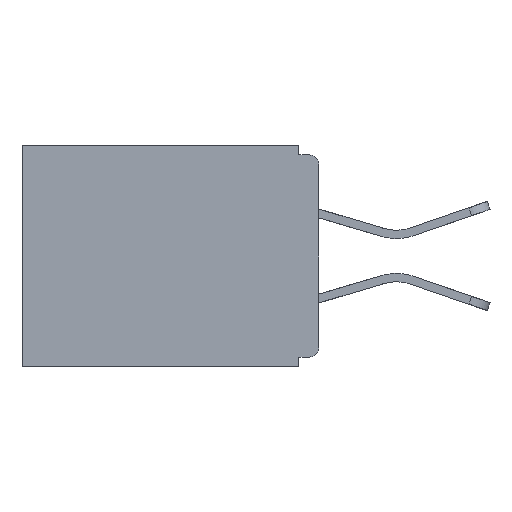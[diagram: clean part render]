
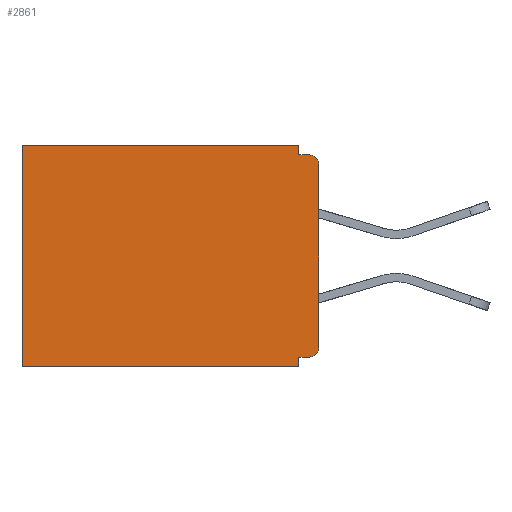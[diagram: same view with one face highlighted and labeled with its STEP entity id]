
A CAD part, left-side view. The second image highlights one B-rep face of the part: STEP entity #2861.
In plain terms, the highlighted planar face has unit normal (-1, 0, 0).
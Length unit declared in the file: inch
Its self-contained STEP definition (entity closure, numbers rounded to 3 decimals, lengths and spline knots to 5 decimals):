
#198 = ORIENTED_EDGE ( 'NONE', *, *, #13432, .T. ) ;
#289 = DIRECTION ( 'NONE',  ( 0., 1., 0. ) ) ;
#593 = AXIS2_PLACEMENT_3D ( 'NONE', #17195, #8387, #11389 ) ;
#1648 = DIRECTION ( 'NONE',  ( 0., 0., -1. ) ) ;
#1740 = ORIENTED_EDGE ( 'NONE', *, *, #16769, .T. ) ;
#2199 = VECTOR ( 'NONE', #4554, 39.37008 ) ;
#2351 = PLANE ( 'NONE',  #15073 ) ;
#2547 = DIRECTION ( 'NONE',  ( 0., 0., -1. ) ) ;
#2598 = EDGE_CURVE ( 'NONE', #16685, #11531, #4499, .T. ) ;
#2722 = ORIENTED_EDGE ( 'NONE', *, *, #9086, .T. ) ;
#2753 = ORIENTED_EDGE ( 'NONE', *, *, #14645, .F. ) ;
#2861 = ADVANCED_FACE ( 'NONE', ( #17775 ), #2351, .F. ) ;
#3551 = EDGE_CURVE ( 'NONE', #8760, #5759, #18661, .T. ) ;
#4011 = VECTOR ( 'NONE', #11175, 39.37008 ) ;
#4232 = EDGE_CURVE ( 'NONE', #6971, #15433, #12115, .T. ) ;
#4321 = VECTOR ( 'NONE', #14092, 39.37008 ) ;
#4493 = CARTESIAN_POINT ( 'NONE',  ( 0.298, 0., -0.328 ) ) ;
#4499 = LINE ( 'NONE', #11701, #15714 ) ;
#4554 = DIRECTION ( 'NONE',  ( 0., -1., 0. ) ) ;
#4942 = CARTESIAN_POINT ( 'NONE',  ( 0.298, 0.46, 0. ) ) ;
#5049 = CARTESIAN_POINT ( 'NONE',  ( 0.298, 0.015, -0.015 ) ) ;
#5377 = CARTESIAN_POINT ( 'NONE',  ( 0.298, 0.031, -0.343 ) ) ;
#5759 = VERTEX_POINT ( 'NONE', #7385 ) ;
#5948 = LINE ( 'NONE', #5377, #7773 ) ;
#6378 = CIRCLE ( 'NONE', #7844, 0.015 ) ;
#6809 = CARTESIAN_POINT ( 'NONE',  ( 0.298, 0., 0. ) ) ;
#6944 = ORIENTED_EDGE ( 'NONE', *, *, #10040, .T. ) ;
#6971 = VERTEX_POINT ( 'NONE', #16929 ) ;
#7042 = ORIENTED_EDGE ( 'NONE', *, *, #14113, .F. ) ;
#7327 = VERTEX_POINT ( 'NONE', #8107 ) ;
#7385 = CARTESIAN_POINT ( 'NONE',  ( 0.298, 0.031, -0.328 ) ) ;
#7593 = CARTESIAN_POINT ( 'NONE',  ( 0.298, 0.46, 0. ) ) ;
#7655 = VECTOR ( 'NONE', #10440, 39.37008 ) ;
#7743 = DIRECTION ( 'NONE',  ( 0., 0., -1. ) ) ;
#7773 = VECTOR ( 'NONE', #8304, 39.37008 ) ;
#7844 = AXIS2_PLACEMENT_3D ( 'NONE', #15994, #16176, #1648 ) ;
#8038 = VECTOR ( 'NONE', #7743, 39.37008 ) ;
#8107 = CARTESIAN_POINT ( 'NONE',  ( 0.298, 0.031, 0. ) ) ;
#8125 = CARTESIAN_POINT ( 'NONE',  ( 0.298, 0., 0. ) ) ;
#8304 = DIRECTION ( 'NONE',  ( 0., 0., -1. ) ) ;
#8387 = DIRECTION ( 'NONE',  ( -1., 0., 0. ) ) ;
#8572 = CARTESIAN_POINT ( 'NONE',  ( 0.298, 0., -0.313 ) ) ;
#8760 = VERTEX_POINT ( 'NONE', #15895 ) ;
#8946 = CARTESIAN_POINT ( 'NONE',  ( 0.298, 0., -0.015 ) ) ;
#9086 = EDGE_CURVE ( 'NONE', #8760, #15433, #6378, .T. ) ;
#9527 = EDGE_LOOP ( 'NONE', ( #6944, #7042, #10122, #198, #1740, #15224, #2753, #11687, #2722, #15324 ) ) ;
#9729 = LINE ( 'NONE', #7593, #7655 ) ;
#9773 = DIRECTION ( 'NONE',  ( 1., 0., 0. ) ) ;
#10040 = EDGE_CURVE ( 'NONE', #6971, #16993, #17358, .T. ) ;
#10122 = ORIENTED_EDGE ( 'NONE', *, *, #10421, .F. ) ;
#10143 = LINE ( 'NONE', #8946, #2199 ) ;
#10421 = EDGE_CURVE ( 'NONE', #7327, #17153, #5948, .T. ) ;
#10440 = DIRECTION ( 'NONE',  ( 0., 0., -1. ) ) ;
#11104 = CARTESIAN_POINT ( 'NONE',  ( 0.298, 0., 0. ) ) ;
#11175 = DIRECTION ( 'NONE',  ( 0., 1., 0. ) ) ;
#11204 = CARTESIAN_POINT ( 'NONE',  ( 0.298, 0.031, -0.015 ) ) ;
#11389 = DIRECTION ( 'NONE',  ( 0., 0., -1. ) ) ;
#11531 = VERTEX_POINT ( 'NONE', #18591 ) ;
#11687 = ORIENTED_EDGE ( 'NONE', *, *, #3551, .F. ) ;
#11701 = CARTESIAN_POINT ( 'NONE',  ( 0.298, 0., -0.343 ) ) ;
#12115 = LINE ( 'NONE', #6809, #4321 ) ;
#13180 = LINE ( 'NONE', #8125, #4011 ) ;
#13349 = DIRECTION ( 'NONE',  ( 0., 1., 0. ) ) ;
#13432 = EDGE_CURVE ( 'NONE', #7327, #16453, #13180, .T. ) ;
#14092 = DIRECTION ( 'NONE',  ( 0., 0., -1. ) ) ;
#14113 = EDGE_CURVE ( 'NONE', #17153, #16993, #10143, .T. ) ;
#14295 = LINE ( 'NONE', #16527, #8038 ) ;
#14645 = EDGE_CURVE ( 'NONE', #5759, #16685, #14295, .T. ) ;
#15073 = AXIS2_PLACEMENT_3D ( 'NONE', #11104, #9773, #2547 ) ;
#15224 = ORIENTED_EDGE ( 'NONE', *, *, #2598, .F. ) ;
#15324 = ORIENTED_EDGE ( 'NONE', *, *, #4232, .F. ) ;
#15433 = VERTEX_POINT ( 'NONE', #8572 ) ;
#15714 = VECTOR ( 'NONE', #289, 39.37008 ) ;
#15895 = CARTESIAN_POINT ( 'NONE',  ( 0.298, 0.015, -0.328 ) ) ;
#15946 = CARTESIAN_POINT ( 'NONE',  ( 0.298, 0.031, -0.343 ) ) ;
#15994 = CARTESIAN_POINT ( 'NONE',  ( 0.298, 0.015, -0.313 ) ) ;
#16176 = DIRECTION ( 'NONE',  ( -1., 0., 0. ) ) ;
#16453 = VERTEX_POINT ( 'NONE', #4942 ) ;
#16527 = CARTESIAN_POINT ( 'NONE',  ( 0.298, 0.031, -0.343 ) ) ;
#16685 = VERTEX_POINT ( 'NONE', #15946 ) ;
#16769 = EDGE_CURVE ( 'NONE', #16453, #11531, #9729, .T. ) ;
#16929 = CARTESIAN_POINT ( 'NONE',  ( 0.298, 0., -0.03 ) ) ;
#16993 = VERTEX_POINT ( 'NONE', #5049 ) ;
#17153 = VERTEX_POINT ( 'NONE', #11204 ) ;
#17195 = CARTESIAN_POINT ( 'NONE',  ( 0.298, 0.015, -0.03 ) ) ;
#17358 = CIRCLE ( 'NONE', #593, 0.015 ) ;
#17775 = FACE_OUTER_BOUND ( 'NONE', #9527, .T. ) ;
#18591 = CARTESIAN_POINT ( 'NONE',  ( 0.298, 0.46, -0.343 ) ) ;
#18661 = LINE ( 'NONE', #4493, #18900 ) ;
#18900 = VECTOR ( 'NONE', #13349, 39.37008 ) ;
